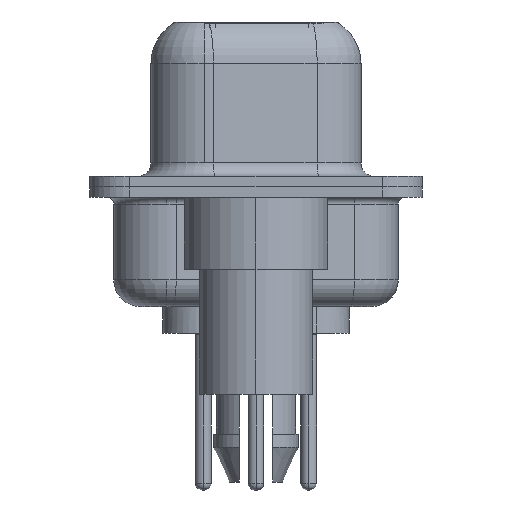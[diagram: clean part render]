
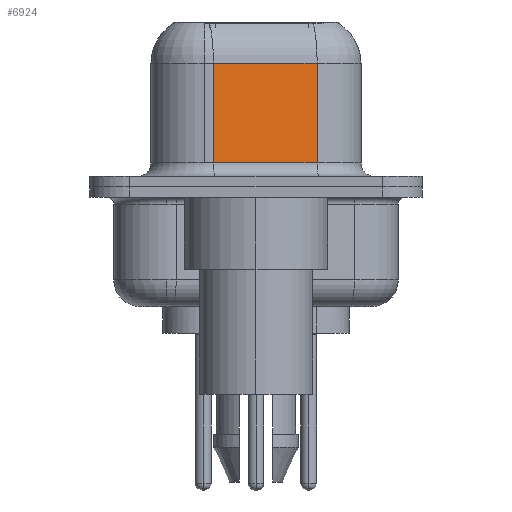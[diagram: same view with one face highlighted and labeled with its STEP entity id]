
A CAD part, left-side view. The second image highlights one B-rep face of the part: STEP entity #6924.
In plain terms, the highlighted planar face has unit normal (-0.985, -0.174, 0).
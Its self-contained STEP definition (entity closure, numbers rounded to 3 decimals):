
#293 = CARTESIAN_POINT ( 'NONE',  ( 5.043, -2.297, 0.9 ) ) ;
#365 = LINE ( 'NONE', #10421, #16432 ) ;
#766 = LINE ( 'NONE', #293, #11421 ) ;
#1967 = EDGE_CURVE ( 'NONE', #29163, #15435, #365, .T. ) ;
#2104 = EDGE_CURVE ( 'NONE', #15435, #2291, #16023, .T. ) ;
#2291 = VERTEX_POINT ( 'NONE', #19359 ) ;
#4015 = EDGE_CURVE ( 'NONE', #2291, #28051, #766, .T. ) ;
#4669 = FACE_OUTER_BOUND ( 'NONE', #25893, .T. ) ;
#4826 = DIRECTION ( 'NONE',  ( -0.174, 0.985, 0. ) ) ;
#5545 = DIRECTION ( 'NONE',  ( 0.174, -0.985, 0. ) ) ;
#6630 = LINE ( 'NONE', #31245, #29128 ) ;
#6924 = ADVANCED_FACE ( 'NONE', ( #4669 ), #17166, .F. ) ;
#8342 = EDGE_CURVE ( 'NONE', #29163, #28051, #6630, .T. ) ;
#8958 = CARTESIAN_POINT ( 'NONE',  ( 4.355, 1.603, 6.4 ) ) ;
#10116 = DIRECTION ( 'NONE',  ( -0.174, 0.985, 0. ) ) ;
#10421 = CARTESIAN_POINT ( 'NONE',  ( 5.043, -2.297, 4.65 ) ) ;
#11328 = VECTOR ( 'NONE', #23030, 1000. ) ;
#11421 = VECTOR ( 'NONE', #5545, 1000. ) ;
#11896 = ORIENTED_EDGE ( 'NONE', *, *, #1967, .T. ) ;
#12211 = DIRECTION ( 'NONE',  ( 0.985, 0.174, 0. ) ) ;
#13403 = CARTESIAN_POINT ( 'NONE',  ( 5.043, -2.297, 4.65 ) ) ;
#15183 = CARTESIAN_POINT ( 'NONE',  ( 4.355, 1.603, 4.65 ) ) ;
#15435 = VERTEX_POINT ( 'NONE', #15183 ) ;
#16023 = LINE ( 'NONE', #8958, #11328 ) ;
#16432 = VECTOR ( 'NONE', #10116, 1000. ) ;
#16462 = ORIENTED_EDGE ( 'NONE', *, *, #4015, .T. ) ;
#17166 = PLANE ( 'NONE',  #18819 ) ;
#17198 = ORIENTED_EDGE ( 'NONE', *, *, #8342, .F. ) ;
#18819 = AXIS2_PLACEMENT_3D ( 'NONE', #19873, #12211, #4826 ) ;
#19359 = CARTESIAN_POINT ( 'NONE',  ( 4.355, 1.603, 0.9 ) ) ;
#19873 = CARTESIAN_POINT ( 'NONE',  ( 5.043, -2.297, 6.4 ) ) ;
#23030 = DIRECTION ( 'NONE',  ( 0., 0., -1. ) ) ;
#23924 = CARTESIAN_POINT ( 'NONE',  ( 5.043, -2.297, 0.9 ) ) ;
#25893 = EDGE_LOOP ( 'NONE', ( #17198, #11896, #29928, #16462 ) ) ;
#28051 = VERTEX_POINT ( 'NONE', #23924 ) ;
#29128 = VECTOR ( 'NONE', #31090, 1000. ) ;
#29163 = VERTEX_POINT ( 'NONE', #13403 ) ;
#29928 = ORIENTED_EDGE ( 'NONE', *, *, #2104, .T. ) ;
#31090 = DIRECTION ( 'NONE',  ( 0., 0., -1. ) ) ;
#31245 = CARTESIAN_POINT ( 'NONE',  ( 5.043, -2.297, 6.4 ) ) ;
